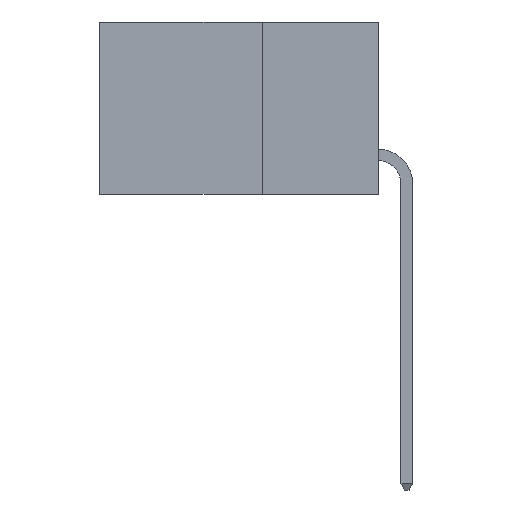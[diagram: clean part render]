
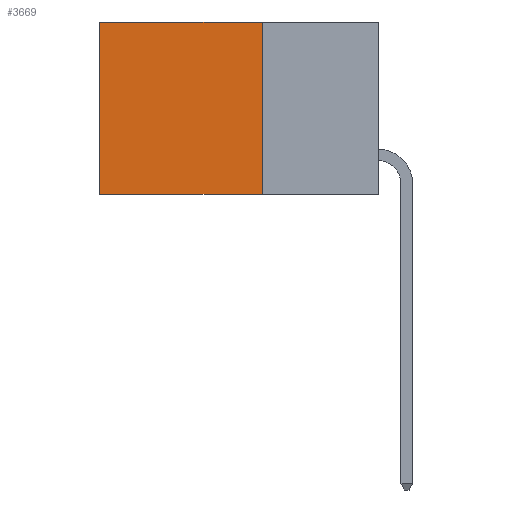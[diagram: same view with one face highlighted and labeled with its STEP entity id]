
A CAD part, left-side view. The second image highlights one B-rep face of the part: STEP entity #3669.
In plain terms, the highlighted planar face has unit normal (-1, 0, 0).
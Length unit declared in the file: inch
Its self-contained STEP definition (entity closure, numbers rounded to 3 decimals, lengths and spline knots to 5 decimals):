
#68 = VECTOR ( 'NONE', #8463, 39.37008 ) ;
#244 = FACE_OUTER_BOUND ( 'NONE', #5457, .T. ) ;
#469 = DIRECTION ( 'NONE',  ( 1., 0., 0. ) ) ;
#1228 = CARTESIAN_POINT ( 'NONE',  ( 0.2615, 0.6, 0. ) ) ;
#2043 = ORIENTED_EDGE ( 'NONE', *, *, #6298, .F. ) ;
#2105 = LINE ( 'NONE', #7374, #3629 ) ;
#2160 = LINE ( 'NONE', #4872, #68 ) ;
#2699 = DIRECTION ( 'NONE',  ( 0., 0., -1. ) ) ;
#2763 = PLANE ( 'NONE',  #3007 ) ;
#2799 = VERTEX_POINT ( 'NONE', #4927 ) ;
#2829 = ORIENTED_EDGE ( 'NONE', *, *, #5592, .T. ) ;
#2999 = VECTOR ( 'NONE', #3098, 39.37008 ) ;
#3007 = AXIS2_PLACEMENT_3D ( 'NONE', #7184, #469, #5772 ) ;
#3098 = DIRECTION ( 'NONE',  ( 0., 1., 0. ) ) ;
#3120 = EDGE_CURVE ( 'NONE', #2799, #9406, #2105, .T. ) ;
#3247 = LINE ( 'NONE', #8861, #2999 ) ;
#3478 = VERTEX_POINT ( 'NONE', #6989 ) ;
#3629 = VECTOR ( 'NONE', #8815, 39.37008 ) ;
#3669 = ADVANCED_FACE ( 'NONE', ( #244 ), #2763, .F. ) ;
#3720 = LINE ( 'NONE', #8521, #5684 ) ;
#4872 = CARTESIAN_POINT ( 'NONE',  ( 0.2615, 0.25, -0.37 ) ) ;
#4927 = CARTESIAN_POINT ( 'NONE',  ( 0.2615, 0.25, 0. ) ) ;
#5457 = EDGE_LOOP ( 'NONE', ( #2829, #2043, #7429, #5986 ) ) ;
#5539 = EDGE_CURVE ( 'NONE', #2799, #3478, #2160, .T. ) ;
#5592 = EDGE_CURVE ( 'NONE', #9406, #7849, #3720, .T. ) ;
#5684 = VECTOR ( 'NONE', #2699, 39.37008 ) ;
#5714 = CARTESIAN_POINT ( 'NONE',  ( 0.2615, 0.6, -0.37 ) ) ;
#5772 = DIRECTION ( 'NONE',  ( 0., 0., -1. ) ) ;
#5986 = ORIENTED_EDGE ( 'NONE', *, *, #3120, .T. ) ;
#6298 = EDGE_CURVE ( 'NONE', #3478, #7849, #3247, .T. ) ;
#6989 = CARTESIAN_POINT ( 'NONE',  ( 0.2615, 0.25, -0.37 ) ) ;
#7184 = CARTESIAN_POINT ( 'NONE',  ( 0.2615, 0.25, -0.37 ) ) ;
#7374 = CARTESIAN_POINT ( 'NONE',  ( 0.2615, 0.25, 0. ) ) ;
#7429 = ORIENTED_EDGE ( 'NONE', *, *, #5539, .F. ) ;
#7849 = VERTEX_POINT ( 'NONE', #5714 ) ;
#8463 = DIRECTION ( 'NONE',  ( 0., 0., -1. ) ) ;
#8521 = CARTESIAN_POINT ( 'NONE',  ( 0.2615, 0.6, -0.37 ) ) ;
#8815 = DIRECTION ( 'NONE',  ( 0., 1., 0. ) ) ;
#8861 = CARTESIAN_POINT ( 'NONE',  ( 0.2615, 0.25, -0.37 ) ) ;
#9406 = VERTEX_POINT ( 'NONE', #1228 ) ;
